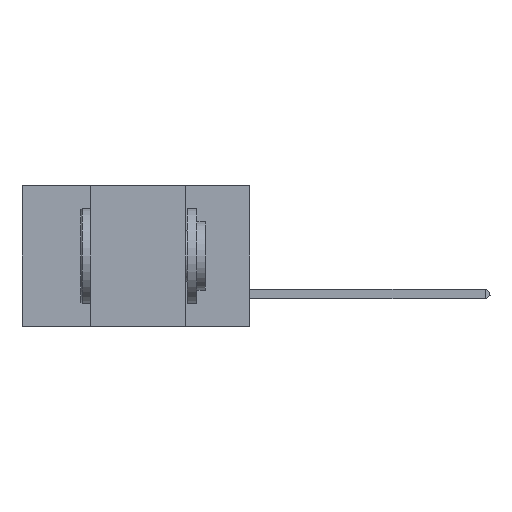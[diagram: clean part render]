
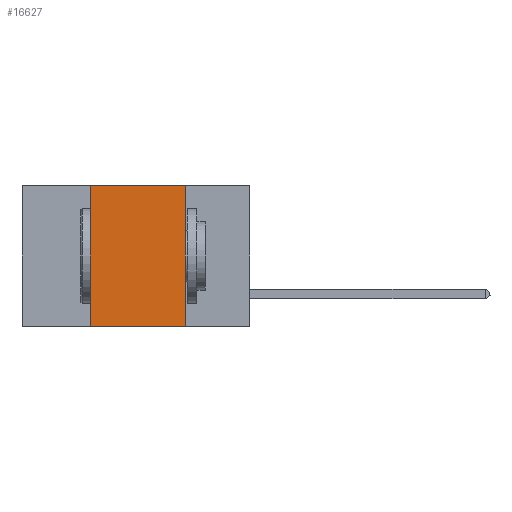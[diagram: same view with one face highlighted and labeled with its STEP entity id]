
A CAD part, left-side view. The second image highlights one B-rep face of the part: STEP entity #16627.
In plain terms, the highlighted planar face has unit normal (-1, 0, 0).
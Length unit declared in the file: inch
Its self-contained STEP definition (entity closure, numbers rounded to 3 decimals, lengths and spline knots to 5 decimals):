
#163 = CARTESIAN_POINT ( 'NONE',  ( 0., 0.6, 0. ) ) ;
#1640 = AXIS2_PLACEMENT_3D ( 'NONE', #163, #16596, #1854 ) ;
#1854 = DIRECTION ( 'NONE',  ( 0., 0., -1. ) ) ;
#1979 = FACE_OUTER_BOUND ( 'NONE', #2296, .T. ) ;
#2108 = VERTEX_POINT ( 'NONE', #5058 ) ;
#2296 = EDGE_LOOP ( 'NONE', ( #5573, #10884, #14919, #4384 ) ) ;
#2909 = VECTOR ( 'NONE', #8756, 39.37008 ) ;
#3395 = LINE ( 'NONE', #16262, #8789 ) ;
#3468 = VERTEX_POINT ( 'NONE', #16967 ) ;
#4384 = ORIENTED_EDGE ( 'NONE', *, *, #14495, .T. ) ;
#4758 = CARTESIAN_POINT ( 'NONE',  ( 0., 0.6, 0. ) ) ;
#5058 = CARTESIAN_POINT ( 'NONE',  ( 0., 0.17, 0. ) ) ;
#5573 = ORIENTED_EDGE ( 'NONE', *, *, #8359, .F. ) ;
#7669 = CARTESIAN_POINT ( 'NONE',  ( 0., 0.42, -0.37 ) ) ;
#8104 = EDGE_CURVE ( 'NONE', #3468, #2108, #16515, .T. ) ;
#8359 = EDGE_CURVE ( 'NONE', #2108, #8458, #19062, .T. ) ;
#8458 = VERTEX_POINT ( 'NONE', #19693 ) ;
#8756 = DIRECTION ( 'NONE',  ( 0., 0., 1. ) ) ;
#8789 = VECTOR ( 'NONE', #17717, 39.37008 ) ;
#9982 = DIRECTION ( 'NONE',  ( 0., 0., -1. ) ) ;
#10682 = VECTOR ( 'NONE', #17574, 39.37008 ) ;
#10884 = ORIENTED_EDGE ( 'NONE', *, *, #8104, .F. ) ;
#12987 = EDGE_CURVE ( 'NONE', #17056, #3468, #14957, .T. ) ;
#13033 = PLANE ( 'NONE',  #1640 ) ;
#14495 = EDGE_CURVE ( 'NONE', #17056, #8458, #3395, .T. ) ;
#14919 = ORIENTED_EDGE ( 'NONE', *, *, #12987, .F. ) ;
#14957 = LINE ( 'NONE', #19891, #2909 ) ;
#16262 = CARTESIAN_POINT ( 'NONE',  ( 0., 0.6, -0.37 ) ) ;
#16515 = LINE ( 'NONE', #4758, #10682 ) ;
#16596 = DIRECTION ( 'NONE',  ( 1., 0., 0. ) ) ;
#16627 = ADVANCED_FACE ( 'NONE', ( #1979 ), #13033, .F. ) ;
#16967 = CARTESIAN_POINT ( 'NONE',  ( 0., 0.42, 0. ) ) ;
#17031 = VECTOR ( 'NONE', #9982, 39.37008 ) ;
#17056 = VERTEX_POINT ( 'NONE', #7669 ) ;
#17574 = DIRECTION ( 'NONE',  ( 0., -1., 0. ) ) ;
#17717 = DIRECTION ( 'NONE',  ( 0., -1., 0. ) ) ;
#19062 = LINE ( 'NONE', #19741, #17031 ) ;
#19693 = CARTESIAN_POINT ( 'NONE',  ( 0., 0.17, -0.37 ) ) ;
#19741 = CARTESIAN_POINT ( 'NONE',  ( 0., 0.17, 0. ) ) ;
#19891 = CARTESIAN_POINT ( 'NONE',  ( 0., 0.42, 0. ) ) ;
